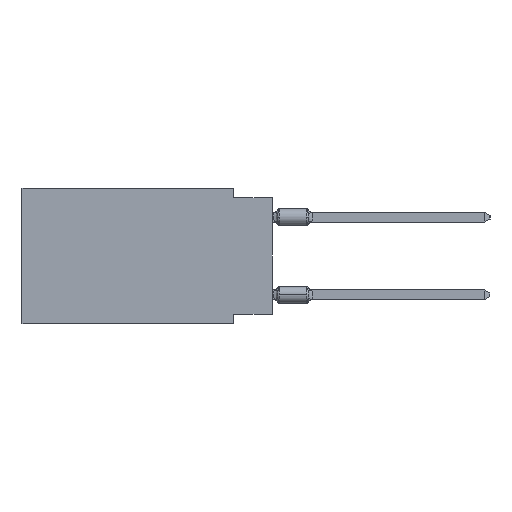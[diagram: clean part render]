
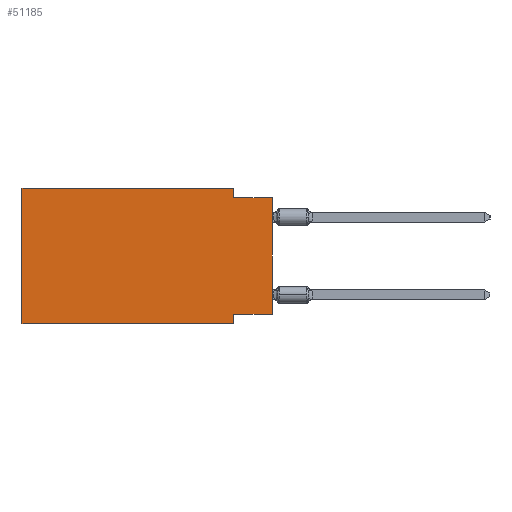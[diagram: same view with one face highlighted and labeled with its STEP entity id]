
A CAD part, left-side view. The second image highlights one B-rep face of the part: STEP entity #51185.
In plain terms, the highlighted planar face has unit normal (-1, 0, 0).
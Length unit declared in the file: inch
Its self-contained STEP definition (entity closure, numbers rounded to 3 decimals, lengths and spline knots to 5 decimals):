
#26 = LINE ( 'NONE', #30469, #16106 ) ;
#450 = VECTOR ( 'NONE', #36431, 39.37008 ) ;
#791 = VERTEX_POINT ( 'NONE', #22927 ) ;
#1272 = LINE ( 'NONE', #35382, #5169 ) ;
#1767 = CARTESIAN_POINT ( 'NONE',  ( 0., 0.645, 0. ) ) ;
#4360 = CARTESIAN_POINT ( 'NONE',  ( 0., 0., -0.025 ) ) ;
#5169 = VECTOR ( 'NONE', #5751, 39.37008 ) ;
#5751 = DIRECTION ( 'NONE',  ( 0., 1., 0. ) ) ;
#6517 = LINE ( 'NONE', #1767, #450 ) ;
#7292 = VERTEX_POINT ( 'NONE', #4360 ) ;
#9066 = VERTEX_POINT ( 'NONE', #39495 ) ;
#9199 = LINE ( 'NONE', #47513, #49784 ) ;
#9551 = VECTOR ( 'NONE', #36208, 39.37008 ) ;
#12662 = EDGE_CURVE ( 'NONE', #9066, #28494, #6517, .T. ) ;
#16106 = VECTOR ( 'NONE', #25743, 39.37008 ) ;
#16763 = ORIENTED_EDGE ( 'NONE', *, *, #30552, .F. ) ;
#17056 = DIRECTION ( 'NONE',  ( 0., -1., 0. ) ) ;
#19846 = FACE_OUTER_BOUND ( 'NONE', #51061, .T. ) ;
#19982 = LINE ( 'NONE', #40400, #9551 ) ;
#21851 = VECTOR ( 'NONE', #42143, 39.37008 ) ;
#22927 = CARTESIAN_POINT ( 'NONE',  ( 0., 0.1, -0.35 ) ) ;
#24759 = ORIENTED_EDGE ( 'NONE', *, *, #45783, .T. ) ;
#24811 = LINE ( 'NONE', #45507, #21851 ) ;
#24871 = CARTESIAN_POINT ( 'NONE',  ( 0., 0.1, -0.35 ) ) ;
#25199 = DIRECTION ( 'NONE',  ( 0., 0., -1. ) ) ;
#25207 = EDGE_CURVE ( 'NONE', #44293, #9066, #24811, .T. ) ;
#25743 = DIRECTION ( 'NONE',  ( 0., -1., 0. ) ) ;
#25786 = CARTESIAN_POINT ( 'NONE',  ( 0., 0.1, -0.325 ) ) ;
#28268 = VERTEX_POINT ( 'NONE', #44165 ) ;
#28494 = VERTEX_POINT ( 'NONE', #54475 ) ;
#29161 = VECTOR ( 'NONE', #25199, 39.37008 ) ;
#29348 = EDGE_CURVE ( 'NONE', #28494, #28268, #32749, .T. ) ;
#30469 = CARTESIAN_POINT ( 'NONE',  ( 0., 0.645, -0.35 ) ) ;
#30552 = EDGE_CURVE ( 'NONE', #28268, #7292, #9199, .T. ) ;
#31475 = ORIENTED_EDGE ( 'NONE', *, *, #41746, .F. ) ;
#32749 = LINE ( 'NONE', #50091, #29161 ) ;
#33879 = ORIENTED_EDGE ( 'NONE', *, *, #40685, .T. ) ;
#34684 = VECTOR ( 'NONE', #45830, 39.37008 ) ;
#35382 = CARTESIAN_POINT ( 'NONE',  ( 0., 0., -0.325 ) ) ;
#36208 = DIRECTION ( 'NONE',  ( 0., 0., 1. ) ) ;
#36431 = DIRECTION ( 'NONE',  ( 0., -1., 0. ) ) ;
#37729 = CARTESIAN_POINT ( 'NONE',  ( 0., 0.645, 0. ) ) ;
#39298 = CARTESIAN_POINT ( 'NONE',  ( 0., 0., -0.325 ) ) ;
#39495 = CARTESIAN_POINT ( 'NONE',  ( 0., 0.645, 0. ) ) ;
#40400 = CARTESIAN_POINT ( 'NONE',  ( 0., 0., 0. ) ) ;
#40685 = EDGE_CURVE ( 'NONE', #50120, #7292, #19982, .T. ) ;
#41379 = DIRECTION ( 'NONE',  ( 1., 0., 0. ) ) ;
#41746 = EDGE_CURVE ( 'NONE', #50120, #52052, #1272, .T. ) ;
#41943 = PLANE ( 'NONE',  #47263 ) ;
#42143 = DIRECTION ( 'NONE',  ( 0., 0., 1. ) ) ;
#42813 = ORIENTED_EDGE ( 'NONE', *, *, #29348, .F. ) ;
#43525 = ORIENTED_EDGE ( 'NONE', *, *, #48544, .F. ) ;
#44165 = CARTESIAN_POINT ( 'NONE',  ( 0., 0.1, -0.025 ) ) ;
#44293 = VERTEX_POINT ( 'NONE', #48978 ) ;
#45507 = CARTESIAN_POINT ( 'NONE',  ( 0., 0.645, 0. ) ) ;
#45783 = EDGE_CURVE ( 'NONE', #44293, #791, #26, .T. ) ;
#45830 = DIRECTION ( 'NONE',  ( 0., 0., -1. ) ) ;
#47263 = AXIS2_PLACEMENT_3D ( 'NONE', #37729, #41379, #54230 ) ;
#47513 = CARTESIAN_POINT ( 'NONE',  ( 0., 0., -0.025 ) ) ;
#48544 = EDGE_CURVE ( 'NONE', #52052, #791, #50038, .T. ) ;
#48978 = CARTESIAN_POINT ( 'NONE',  ( 0., 0.645, -0.35 ) ) ;
#49161 = ORIENTED_EDGE ( 'NONE', *, *, #12662, .F. ) ;
#49784 = VECTOR ( 'NONE', #17056, 39.37008 ) ;
#50038 = LINE ( 'NONE', #24871, #34684 ) ;
#50091 = CARTESIAN_POINT ( 'NONE',  ( 0., 0.1, 0. ) ) ;
#50120 = VERTEX_POINT ( 'NONE', #39298 ) ;
#51061 = EDGE_LOOP ( 'NONE', ( #33879, #16763, #42813, #49161, #51397, #24759, #43525, #31475 ) ) ;
#51185 = ADVANCED_FACE ( 'NONE', ( #19846 ), #41943, .F. ) ;
#51397 = ORIENTED_EDGE ( 'NONE', *, *, #25207, .F. ) ;
#52052 = VERTEX_POINT ( 'NONE', #25786 ) ;
#54230 = DIRECTION ( 'NONE',  ( 0., 0., -1. ) ) ;
#54475 = CARTESIAN_POINT ( 'NONE',  ( 0., 0.1, 0. ) ) ;
